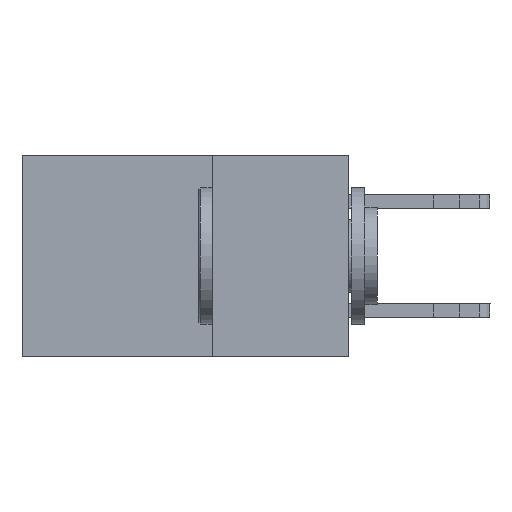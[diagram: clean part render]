
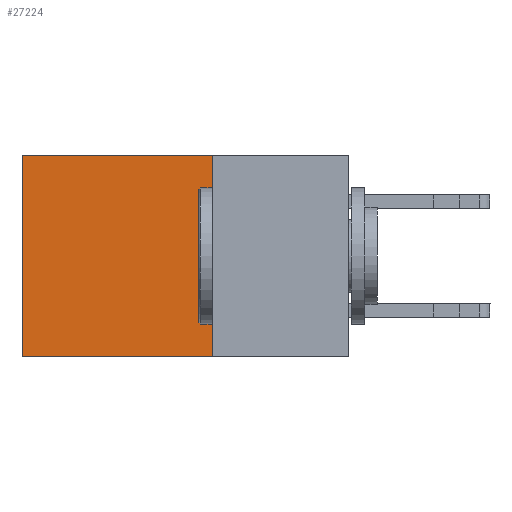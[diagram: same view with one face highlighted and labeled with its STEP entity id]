
A CAD part, left-side view. The second image highlights one B-rep face of the part: STEP entity #27224.
In plain terms, the highlighted planar face has unit normal (-1, 0, 0).
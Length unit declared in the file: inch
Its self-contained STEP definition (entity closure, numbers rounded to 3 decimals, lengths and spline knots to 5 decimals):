
#823 = CARTESIAN_POINT ( 'NONE',  ( 0.298, 0.6, -0.37 ) ) ;
#912 = DIRECTION ( 'NONE',  ( 0., 0., -1. ) ) ;
#1007 = PLANE ( 'NONE',  #16391 ) ;
#1385 = EDGE_CURVE ( 'NONE', #24625, #10090, #8043, .T. ) ;
#2485 = VECTOR ( 'NONE', #27041, 39.37008 ) ;
#2575 = ORIENTED_EDGE ( 'NONE', *, *, #10254, .T. ) ;
#2714 = ORIENTED_EDGE ( 'NONE', *, *, #1385, .T. ) ;
#3517 = EDGE_CURVE ( 'NONE', #24625, #5710, #24997, .T. ) ;
#4176 = VECTOR ( 'NONE', #10206, 39.37008 ) ;
#5710 = VERTEX_POINT ( 'NONE', #27166 ) ;
#7144 = DIRECTION ( 'NONE',  ( 1., 0., 0. ) ) ;
#7412 = CARTESIAN_POINT ( 'NONE',  ( 0.298, 0.25, 0. ) ) ;
#8043 = LINE ( 'NONE', #24758, #2485 ) ;
#9374 = DIRECTION ( 'NONE',  ( 0., 0., -1. ) ) ;
#9818 = VECTOR ( 'NONE', #9374, 39.37008 ) ;
#10090 = VERTEX_POINT ( 'NONE', #19632 ) ;
#10206 = DIRECTION ( 'NONE',  ( 0., 1., 0. ) ) ;
#10254 = EDGE_CURVE ( 'NONE', #10090, #19490, #15427, .T. ) ;
#11304 = EDGE_CURVE ( 'NONE', #5710, #19490, #12404, .T. ) ;
#11340 = CARTESIAN_POINT ( 'NONE',  ( 0.298, 0.25, 0. ) ) ;
#11367 = ORIENTED_EDGE ( 'NONE', *, *, #3517, .F. ) ;
#12404 = LINE ( 'NONE', #22885, #4176 ) ;
#15427 = LINE ( 'NONE', #26237, #9818 ) ;
#15693 = DIRECTION ( 'NONE',  ( 0., 0., -1. ) ) ;
#16391 = AXIS2_PLACEMENT_3D ( 'NONE', #7412, #7144, #15693 ) ;
#19067 = EDGE_LOOP ( 'NONE', ( #2575, #21883, #11367, #2714 ) ) ;
#19490 = VERTEX_POINT ( 'NONE', #823 ) ;
#19632 = CARTESIAN_POINT ( 'NONE',  ( 0.298, 0.6, 0. ) ) ;
#19999 = VECTOR ( 'NONE', #912, 39.37008 ) ;
#20293 = FACE_OUTER_BOUND ( 'NONE', #19067, .T. ) ;
#21883 = ORIENTED_EDGE ( 'NONE', *, *, #11304, .F. ) ;
#22885 = CARTESIAN_POINT ( 'NONE',  ( 0.298, 0.25, -0.37 ) ) ;
#23788 = CARTESIAN_POINT ( 'NONE',  ( 0.298, 0.25, 0. ) ) ;
#24625 = VERTEX_POINT ( 'NONE', #23788 ) ;
#24758 = CARTESIAN_POINT ( 'NONE',  ( 0.298, 0.25, 0. ) ) ;
#24997 = LINE ( 'NONE', #11340, #19999 ) ;
#26237 = CARTESIAN_POINT ( 'NONE',  ( 0.298, 0.6, 0. ) ) ;
#27041 = DIRECTION ( 'NONE',  ( 0., 1., 0. ) ) ;
#27166 = CARTESIAN_POINT ( 'NONE',  ( 0.298, 0.25, -0.37 ) ) ;
#27224 = ADVANCED_FACE ( 'NONE', ( #20293 ), #1007, .F. ) ;
